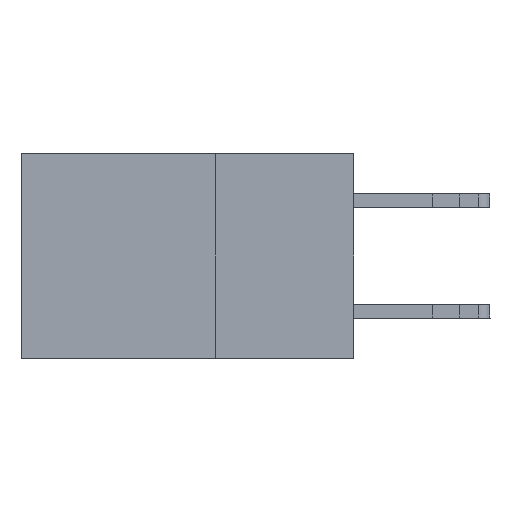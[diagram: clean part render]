
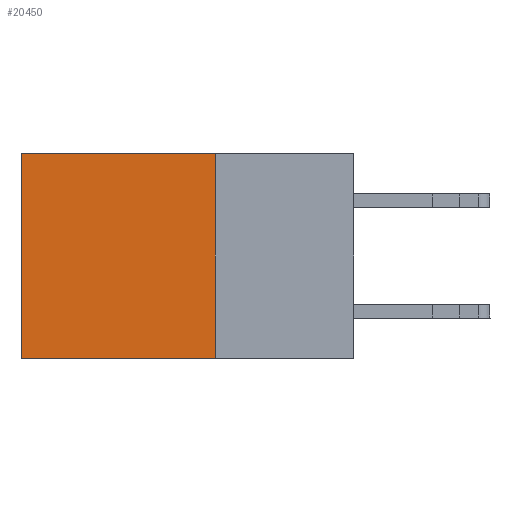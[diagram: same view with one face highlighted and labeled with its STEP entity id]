
A CAD part, left-side view. The second image highlights one B-rep face of the part: STEP entity #20450.
In plain terms, the highlighted planar face has unit normal (-1, 0, 0).
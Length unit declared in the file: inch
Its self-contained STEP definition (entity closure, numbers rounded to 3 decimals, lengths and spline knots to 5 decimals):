
#166 = LINE ( 'NONE', #5392, #18347 ) ;
#379 = LINE ( 'NONE', #17327, #17544 ) ;
#637 = LINE ( 'NONE', #20867, #16323 ) ;
#1624 = CARTESIAN_POINT ( 'NONE',  ( 0.2875, 0.25, 0. ) ) ;
#2143 = LINE ( 'NONE', #5778, #12751 ) ;
#2515 = CARTESIAN_POINT ( 'NONE',  ( 0.2875, 0.6, -0.37 ) ) ;
#2899 = ORIENTED_EDGE ( 'NONE', *, *, #16934, .F. ) ;
#2952 = EDGE_CURVE ( 'NONE', #10867, #12130, #166, .T. ) ;
#3507 = EDGE_CURVE ( 'NONE', #10176, #10867, #637, .T. ) ;
#4860 = DIRECTION ( 'NONE',  ( 0., 0., -1. ) ) ;
#5392 = CARTESIAN_POINT ( 'NONE',  ( 0.2875, 0.6, 0. ) ) ;
#5778 = CARTESIAN_POINT ( 'NONE',  ( 0.2875, 0.25, 0. ) ) ;
#6502 = CARTESIAN_POINT ( 'NONE',  ( 0.2875, 0.6, 0. ) ) ;
#6918 = DIRECTION ( 'NONE',  ( 0., 0., -1. ) ) ;
#7392 = DIRECTION ( 'NONE',  ( 0., 1., 0. ) ) ;
#7569 = DIRECTION ( 'NONE',  ( 0., 1., 0. ) ) ;
#10176 = VERTEX_POINT ( 'NONE', #11384 ) ;
#10707 = ORIENTED_EDGE ( 'NONE', *, *, #14248, .F. ) ;
#10867 = VERTEX_POINT ( 'NONE', #6502 ) ;
#11206 = CARTESIAN_POINT ( 'NONE',  ( 0.2875, 0.25, -0.37 ) ) ;
#11384 = CARTESIAN_POINT ( 'NONE',  ( 0.2875, 0.25, 0. ) ) ;
#12130 = VERTEX_POINT ( 'NONE', #2515 ) ;
#12751 = VECTOR ( 'NONE', #19065, 39.37008 ) ;
#12990 = AXIS2_PLACEMENT_3D ( 'NONE', #1624, #15132, #4860 ) ;
#14248 = EDGE_CURVE ( 'NONE', #10176, #15076, #2143, .T. ) ;
#14911 = FACE_OUTER_BOUND ( 'NONE', #15732, .T. ) ;
#15076 = VERTEX_POINT ( 'NONE', #11206 ) ;
#15132 = DIRECTION ( 'NONE',  ( 1., 0., 0. ) ) ;
#15732 = EDGE_LOOP ( 'NONE', ( #17041, #2899, #10707, #20291 ) ) ;
#16323 = VECTOR ( 'NONE', #7392, 39.37008 ) ;
#16833 = PLANE ( 'NONE',  #12990 ) ;
#16934 = EDGE_CURVE ( 'NONE', #15076, #12130, #379, .T. ) ;
#17041 = ORIENTED_EDGE ( 'NONE', *, *, #2952, .T. ) ;
#17327 = CARTESIAN_POINT ( 'NONE',  ( 0.2875, 0.25, -0.37 ) ) ;
#17544 = VECTOR ( 'NONE', #7569, 39.37008 ) ;
#18347 = VECTOR ( 'NONE', #6918, 39.37008 ) ;
#19065 = DIRECTION ( 'NONE',  ( 0., 0., -1. ) ) ;
#20291 = ORIENTED_EDGE ( 'NONE', *, *, #3507, .T. ) ;
#20450 = ADVANCED_FACE ( 'NONE', ( #14911 ), #16833, .F. ) ;
#20867 = CARTESIAN_POINT ( 'NONE',  ( 0.2875, 0.25, 0. ) ) ;
